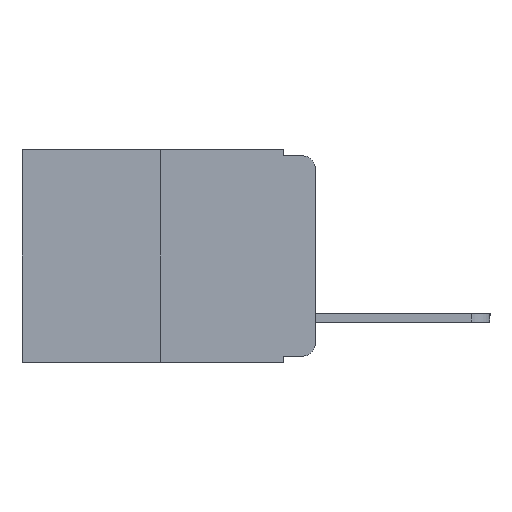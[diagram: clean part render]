
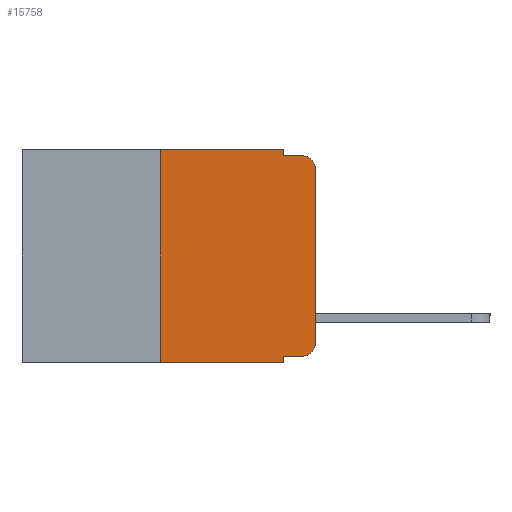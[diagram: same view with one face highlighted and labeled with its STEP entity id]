
A CAD part, left-side view. The second image highlights one B-rep face of the part: STEP entity #15758.
In plain terms, the highlighted planar face has unit normal (-1, 0, 0).
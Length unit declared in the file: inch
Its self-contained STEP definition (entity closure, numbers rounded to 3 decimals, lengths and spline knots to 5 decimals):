
#33 = CARTESIAN_POINT ( 'NONE',  ( 0., 0.051, -0.01 ) ) ;
#149 = LINE ( 'NONE', #16133, #12982 ) ;
#732 = DIRECTION ( 'NONE',  ( 0., -1., 0. ) ) ;
#870 = PLANE ( 'NONE',  #11773 ) ;
#1019 = DIRECTION ( 'NONE',  ( 0., 0., -1. ) ) ;
#1233 = VERTEX_POINT ( 'NONE', #5203 ) ;
#1560 = CARTESIAN_POINT ( 'NONE',  ( 0., 0.25, 0. ) ) ;
#1794 = DIRECTION ( 'NONE',  ( 0., -1., 0. ) ) ;
#2258 = DIRECTION ( 'NONE',  ( 0., 0., 1. ) ) ;
#2450 = CARTESIAN_POINT ( 'NONE',  ( 0., 0.473, -0.343 ) ) ;
#2522 = CARTESIAN_POINT ( 'NONE',  ( 0., 0.051, -0.333 ) ) ;
#2587 = DIRECTION ( 'NONE',  ( 1., 0., 0. ) ) ;
#2621 = DIRECTION ( 'NONE',  ( -1., 0., 0. ) ) ;
#2725 = EDGE_CURVE ( 'NONE', #19339, #1233, #149, .T. ) ;
#3413 = VECTOR ( 'NONE', #1794, 39.37008 ) ;
#3588 = CARTESIAN_POINT ( 'NONE',  ( 0., 0.051, 0. ) ) ;
#3894 = DIRECTION ( 'NONE',  ( 0., -1., 0. ) ) ;
#5151 = VERTEX_POINT ( 'NONE', #13522 ) ;
#5203 = CARTESIAN_POINT ( 'NONE',  ( 0., 0.051, -0.343 ) ) ;
#5417 = AXIS2_PLACEMENT_3D ( 'NONE', #12570, #2621, #14259 ) ;
#6144 = EDGE_CURVE ( 'NONE', #14867, #10692, #9962, .T. ) ;
#6148 = VERTEX_POINT ( 'NONE', #10993 ) ;
#6280 = LINE ( 'NONE', #12160, #10693 ) ;
#6376 = FACE_OUTER_BOUND ( 'NONE', #19972, .T. ) ;
#6608 = CIRCLE ( 'NONE', #5417, 0.02 ) ;
#7124 = CARTESIAN_POINT ( 'NONE',  ( 0., 0., 0. ) ) ;
#7622 = CARTESIAN_POINT ( 'NONE',  ( 0., 0.02, -0.313 ) ) ;
#7849 = LINE ( 'NONE', #33, #3413 ) ;
#8081 = DIRECTION ( 'NONE',  ( 0., -1., 0. ) ) ;
#8675 = DIRECTION ( 'NONE',  ( 0., 0., 1. ) ) ;
#8849 = CIRCLE ( 'NONE', #18010, 0.02 ) ;
#8994 = EDGE_CURVE ( 'NONE', #13315, #11423, #6608, .T. ) ;
#9242 = DIRECTION ( 'NONE',  ( 0., 0., -1. ) ) ;
#9274 = CARTESIAN_POINT ( 'NONE',  ( 0., 0.051, -0.01 ) ) ;
#9701 = VECTOR ( 'NONE', #2258, 39.37008 ) ;
#9962 = LINE ( 'NONE', #20852, #18307 ) ;
#9981 = EDGE_CURVE ( 'NONE', #6148, #13315, #13286, .T. ) ;
#10554 = CARTESIAN_POINT ( 'NONE',  ( 0., 0.25, 0. ) ) ;
#10692 = VERTEX_POINT ( 'NONE', #9274 ) ;
#10693 = VECTOR ( 'NONE', #3894, 39.37008 ) ;
#10856 = CARTESIAN_POINT ( 'NONE',  ( 0., 0.473, 0. ) ) ;
#10861 = EDGE_CURVE ( 'NONE', #19339, #14621, #13247, .T. ) ;
#10993 = CARTESIAN_POINT ( 'NONE',  ( 0., 0., -0.313 ) ) ;
#11046 = VERTEX_POINT ( 'NONE', #1560 ) ;
#11332 = EDGE_CURVE ( 'NONE', #5151, #1233, #16662, .T. ) ;
#11423 = VERTEX_POINT ( 'NONE', #20805 ) ;
#11773 = AXIS2_PLACEMENT_3D ( 'NONE', #10856, #2587, #14232 ) ;
#11985 = EDGE_CURVE ( 'NONE', #14621, #6148, #8849, .T. ) ;
#12160 = CARTESIAN_POINT ( 'NONE',  ( 0., 0.473, 0. ) ) ;
#12570 = CARTESIAN_POINT ( 'NONE',  ( 0., 0.02, -0.03 ) ) ;
#12982 = VECTOR ( 'NONE', #16659, 39.37008 ) ;
#13247 = LINE ( 'NONE', #16368, #21437 ) ;
#13286 = LINE ( 'NONE', #7124, #17749 ) ;
#13315 = VERTEX_POINT ( 'NONE', #17365 ) ;
#13373 = ORIENTED_EDGE ( 'NONE', *, *, #11985, .T. ) ;
#13522 = CARTESIAN_POINT ( 'NONE',  ( 0., 0.25, -0.343 ) ) ;
#14232 = DIRECTION ( 'NONE',  ( 0., 0., -1. ) ) ;
#14259 = DIRECTION ( 'NONE',  ( 0., 0., -1. ) ) ;
#14621 = VERTEX_POINT ( 'NONE', #19314 ) ;
#14867 = VERTEX_POINT ( 'NONE', #3588 ) ;
#15740 = ORIENTED_EDGE ( 'NONE', *, *, #2725, .F. ) ;
#15758 = ADVANCED_FACE ( 'NONE', ( #6376 ), #870, .F. ) ;
#16133 = CARTESIAN_POINT ( 'NONE',  ( 0., 0.051, 0. ) ) ;
#16256 = ORIENTED_EDGE ( 'NONE', *, *, #10861, .T. ) ;
#16274 = EDGE_CURVE ( 'NONE', #5151, #11046, #19064, .T. ) ;
#16368 = CARTESIAN_POINT ( 'NONE',  ( 0., 0.051, -0.333 ) ) ;
#16479 = ORIENTED_EDGE ( 'NONE', *, *, #9981, .T. ) ;
#16659 = DIRECTION ( 'NONE',  ( 0., 0., -1. ) ) ;
#16662 = LINE ( 'NONE', #2450, #20913 ) ;
#17025 = ORIENTED_EDGE ( 'NONE', *, *, #8994, .T. ) ;
#17281 = ORIENTED_EDGE ( 'NONE', *, *, #18003, .F. ) ;
#17365 = CARTESIAN_POINT ( 'NONE',  ( 0., 0., -0.03 ) ) ;
#17749 = VECTOR ( 'NONE', #8675, 39.37008 ) ;
#18003 = EDGE_CURVE ( 'NONE', #11046, #14867, #6280, .T. ) ;
#18010 = AXIS2_PLACEMENT_3D ( 'NONE', #7622, #19180, #9242 ) ;
#18307 = VECTOR ( 'NONE', #1019, 39.37008 ) ;
#19025 = ORIENTED_EDGE ( 'NONE', *, *, #21007, .F. ) ;
#19060 = ORIENTED_EDGE ( 'NONE', *, *, #11332, .T. ) ;
#19064 = LINE ( 'NONE', #10554, #9701 ) ;
#19180 = DIRECTION ( 'NONE',  ( -1., 0., 0. ) ) ;
#19314 = CARTESIAN_POINT ( 'NONE',  ( 0., 0.02, -0.333 ) ) ;
#19339 = VERTEX_POINT ( 'NONE', #2522 ) ;
#19972 = EDGE_LOOP ( 'NONE', ( #16479, #17025, #19025, #21015, #17281, #21277, #19060, #15740, #16256, #13373 ) ) ;
#20805 = CARTESIAN_POINT ( 'NONE',  ( 0., 0.02, -0.01 ) ) ;
#20852 = CARTESIAN_POINT ( 'NONE',  ( 0., 0.051, 0. ) ) ;
#20913 = VECTOR ( 'NONE', #732, 39.37008 ) ;
#21007 = EDGE_CURVE ( 'NONE', #10692, #11423, #7849, .T. ) ;
#21015 = ORIENTED_EDGE ( 'NONE', *, *, #6144, .F. ) ;
#21277 = ORIENTED_EDGE ( 'NONE', *, *, #16274, .F. ) ;
#21437 = VECTOR ( 'NONE', #8081, 39.37008 ) ;
